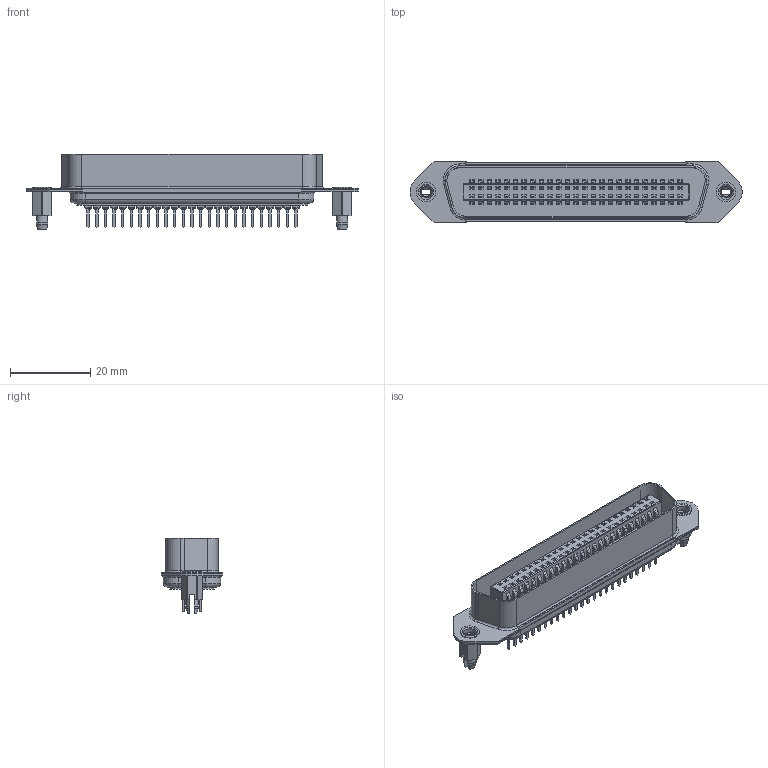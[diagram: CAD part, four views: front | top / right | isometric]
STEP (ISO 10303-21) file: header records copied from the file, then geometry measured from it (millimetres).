
FILE_DESCRIPTION (( 'STEP AP203' ), '1' );
FILE_NAME ('B57-150-621-802.STEP', '2020-06-24T12:36:27', ( '' ), ( '' ), 'SwSTEP 2.0', 'SolidWorks 2020', '' );
FILE_SCHEMA (( 'CONFIG_CONTROL_DESIGN' ));
Length unit declared in the file: millimetre
Products named in the file (6): B57 Housing Insert MALE_50 Position UP; B57-150-621-802; B57 Contacts MALE_50 Position STR; B57 Rivet_STR THREAD BOARDLOCK ; B57 Back Shell_50 Position; B57 Front Shell MALE_50 Position UP
Assembly tree (6 placements, depth 2):
  B57-150-621-802
    B57 Back Shell_50 Position
    B57 Rivet_STR THREAD BOARDLOCK   x2
    B57 Housing Insert MALE_50 Position UP
    B57 Front Shell MALE_50 Position UP
    B57 Contacts MALE_50 Position STR
Bounding box: 82.83 x 15.3 x 18.8 mm (x, y, z)
Volume: 6003.2 mm3; surface area: 14647.9 mm2
Topology: 55 solids, 55 shells, 4943 faces, 14011 edges, 8880 vertices
Faces by surface type: plane 3430, cylinder 1255, sphere 204, torus 30, cone 14, bspline 10
Entity records: 158200 total; most frequent: CARTESIAN_POINT 31844, ORIENTED_EDGE 27240, DIRECTION 24945, EDGE_CURVE 13620, VECTOR 10885, LINE 10885, VERTEX_POINT 8756, AXIS2_PLACEMENT_3D 7030
